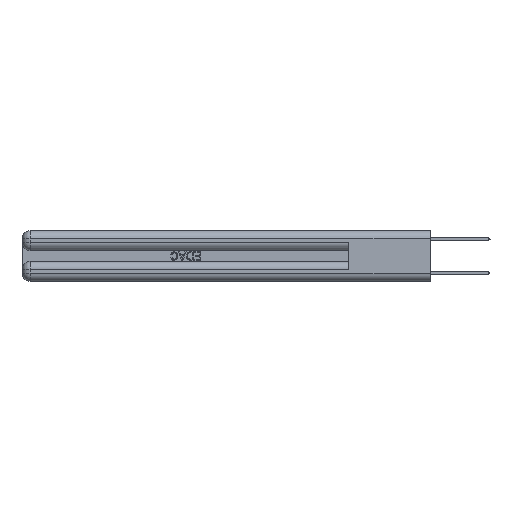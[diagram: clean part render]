
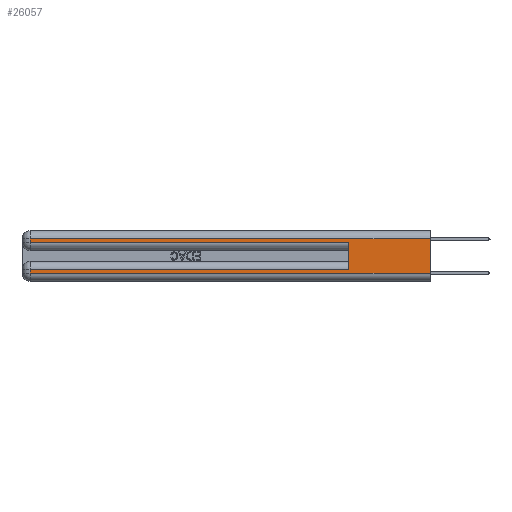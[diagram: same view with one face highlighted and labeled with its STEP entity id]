
A CAD part, left-side view. The second image highlights one B-rep face of the part: STEP entity #26057.
In plain terms, the highlighted planar face has unit normal (-1, 0, 0).
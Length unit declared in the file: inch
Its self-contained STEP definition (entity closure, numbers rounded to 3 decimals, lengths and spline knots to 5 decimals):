
#206 = EDGE_LOOP ( 'NONE', ( #24872, #6027, #24296, #12997, #19143, #10717, #24029, #23541 ) ) ;
#384 = CARTESIAN_POINT ( 'NONE',  ( 0., 0., 0.37 ) ) ;
#2089 = DIRECTION ( 'NONE',  ( 0., 0., -1. ) ) ;
#2157 = VERTEX_POINT ( 'NONE', #21856 ) ;
#2792 = LINE ( 'NONE', #15565, #11649 ) ;
#3312 = CARTESIAN_POINT ( 'NONE',  ( 0., 0., 0.31 ) ) ;
#3673 = DIRECTION ( 'NONE',  ( 0., 0., -1. ) ) ;
#3949 = DIRECTION ( 'NONE',  ( 0., 0., 1. ) ) ;
#4006 = VECTOR ( 'NONE', #8465, 39.37008 ) ;
#5084 = EDGE_CURVE ( 'NONE', #16979, #13732, #30202, .T. ) ;
#6027 = ORIENTED_EDGE ( 'NONE', *, *, #23959, .T. ) ;
#6513 = VERTEX_POINT ( 'NONE', #27305 ) ;
#6969 = CARTESIAN_POINT ( 'NONE',  ( 0., 2.94, 0.37 ) ) ;
#7544 = LINE ( 'NONE', #29262, #21203 ) ;
#7555 = VECTOR ( 'NONE', #11145, 39.37008 ) ;
#8465 = DIRECTION ( 'NONE',  ( 0., 1., 0. ) ) ;
#8831 = CARTESIAN_POINT ( 'NONE',  ( 0., 0., 0.06 ) ) ;
#9831 = LINE ( 'NONE', #6969, #15749 ) ;
#10465 = VERTEX_POINT ( 'NONE', #29287 ) ;
#10717 = ORIENTED_EDGE ( 'NONE', *, *, #28257, .T. ) ;
#11126 = VERTEX_POINT ( 'NONE', #3312 ) ;
#11145 = DIRECTION ( 'NONE',  ( 0., 1., 0. ) ) ;
#11516 = EDGE_CURVE ( 'NONE', #26992, #6513, #17403, .T. ) ;
#11646 = CARTESIAN_POINT ( 'NONE',  ( 0., 0.6, 0.285 ) ) ;
#11649 = VECTOR ( 'NONE', #3949, 39.37008 ) ;
#12677 = CARTESIAN_POINT ( 'NONE',  ( 0., 0., 0.285 ) ) ;
#12997 = ORIENTED_EDGE ( 'NONE', *, *, #5084, .T. ) ;
#13732 = VERTEX_POINT ( 'NONE', #11646 ) ;
#13826 = LINE ( 'NONE', #30000, #7555 ) ;
#15565 = CARTESIAN_POINT ( 'NONE',  ( 0., 0.6, 0.145 ) ) ;
#15629 = CARTESIAN_POINT ( 'NONE',  ( 0., 2.94, 0.285 ) ) ;
#15749 = VECTOR ( 'NONE', #2089, 39.37008 ) ;
#15785 = CARTESIAN_POINT ( 'NONE',  ( 0., 0., 0.37 ) ) ;
#15883 = DIRECTION ( 'NONE',  ( 1., 0., 0. ) ) ;
#16979 = VERTEX_POINT ( 'NONE', #15629 ) ;
#17403 = LINE ( 'NONE', #8831, #20699 ) ;
#17606 = CARTESIAN_POINT ( 'NONE',  ( 0., 2.94, 0.06 ) ) ;
#17967 = CARTESIAN_POINT ( 'NONE',  ( 0., 0., 0.085 ) ) ;
#18864 = FACE_OUTER_BOUND ( 'NONE', #206, .T. ) ;
#19018 = DIRECTION ( 'NONE',  ( 0., 0., -1. ) ) ;
#19143 = ORIENTED_EDGE ( 'NONE', *, *, #30526, .F. ) ;
#19626 = EDGE_CURVE ( 'NONE', #11126, #6513, #25993, .T. ) ;
#20474 = EDGE_CURVE ( 'NONE', #10465, #26992, #7544, .T. ) ;
#20478 = VECTOR ( 'NONE', #19018, 39.37008 ) ;
#20699 = VECTOR ( 'NONE', #25238, 39.37008 ) ;
#21133 = EDGE_CURVE ( 'NONE', #23937, #16979, #9831, .T. ) ;
#21203 = VECTOR ( 'NONE', #24737, 39.37008 ) ;
#21550 = AXIS2_PLACEMENT_3D ( 'NONE', #15785, #15883, #3673 ) ;
#21856 = CARTESIAN_POINT ( 'NONE',  ( 0., 0.6, 0.085 ) ) ;
#23541 = ORIENTED_EDGE ( 'NONE', *, *, #11516, .T. ) ;
#23937 = VERTEX_POINT ( 'NONE', #29498 ) ;
#23959 = EDGE_CURVE ( 'NONE', #11126, #23937, #13826, .T. ) ;
#23963 = VECTOR ( 'NONE', #25057, 39.37008 ) ;
#24029 = ORIENTED_EDGE ( 'NONE', *, *, #20474, .T. ) ;
#24296 = ORIENTED_EDGE ( 'NONE', *, *, #21133, .T. ) ;
#24737 = DIRECTION ( 'NONE',  ( 0., 0., -1. ) ) ;
#24850 = PLANE ( 'NONE',  #21550 ) ;
#24872 = ORIENTED_EDGE ( 'NONE', *, *, #19626, .F. ) ;
#25057 = DIRECTION ( 'NONE',  ( 0., -1., 0. ) ) ;
#25238 = DIRECTION ( 'NONE',  ( 0., -1., 0. ) ) ;
#25450 = LINE ( 'NONE', #17967, #4006 ) ;
#25993 = LINE ( 'NONE', #384, #20478 ) ;
#26057 = ADVANCED_FACE ( 'NONE', ( #18864 ), #24850, .F. ) ;
#26992 = VERTEX_POINT ( 'NONE', #17606 ) ;
#27305 = CARTESIAN_POINT ( 'NONE',  ( 0., 0., 0.06 ) ) ;
#28257 = EDGE_CURVE ( 'NONE', #2157, #10465, #25450, .T. ) ;
#29262 = CARTESIAN_POINT ( 'NONE',  ( 0., 2.94, 0.37 ) ) ;
#29287 = CARTESIAN_POINT ( 'NONE',  ( 0., 2.94, 0.085 ) ) ;
#29498 = CARTESIAN_POINT ( 'NONE',  ( 0., 2.94, 0.31 ) ) ;
#30000 = CARTESIAN_POINT ( 'NONE',  ( 0., 0., 0.31 ) ) ;
#30202 = LINE ( 'NONE', #12677, #23963 ) ;
#30526 = EDGE_CURVE ( 'NONE', #2157, #13732, #2792, .T. ) ;
